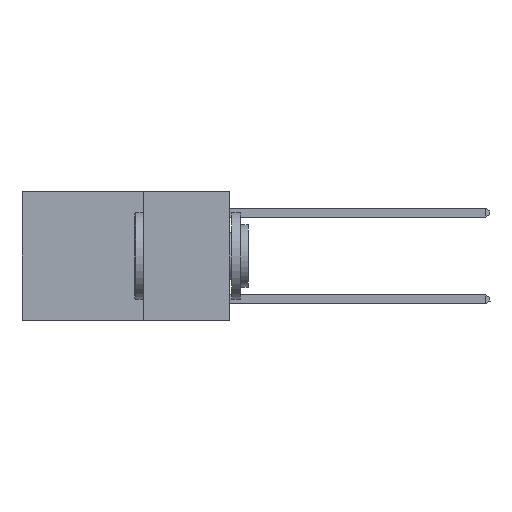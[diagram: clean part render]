
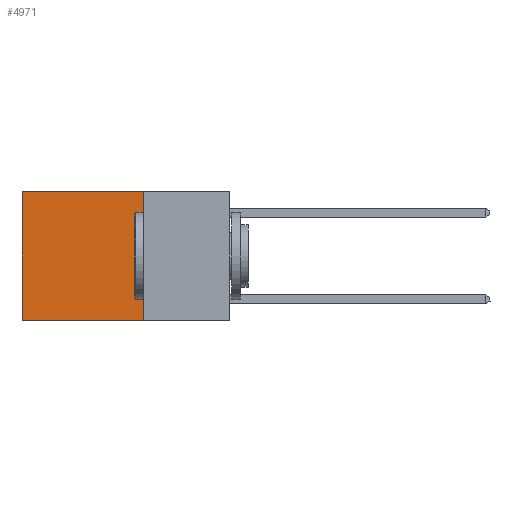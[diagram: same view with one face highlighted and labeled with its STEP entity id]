
A CAD part, left-side view. The second image highlights one B-rep face of the part: STEP entity #4971.
In plain terms, the highlighted planar face has unit normal (-1, 0, 0).
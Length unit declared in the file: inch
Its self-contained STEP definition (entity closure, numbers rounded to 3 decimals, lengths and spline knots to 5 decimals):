
#1460 = LINE ( 'NONE', #19695, #10161 ) ;
#1607 = CARTESIAN_POINT ( 'NONE',  ( 0.2625, 0.6, 0. ) ) ;
#2609 = DIRECTION ( 'NONE',  ( 1., 0., 0. ) ) ;
#2805 = VERTEX_POINT ( 'NONE', #18746 ) ;
#3297 = CARTESIAN_POINT ( 'NONE',  ( 0.2625, 0.25, -0.37 ) ) ;
#4663 = ORIENTED_EDGE ( 'NONE', *, *, #7768, .F. ) ;
#4971 = ADVANCED_FACE ( 'NONE', ( #6856 ), #11848, .F. ) ;
#6209 = CARTESIAN_POINT ( 'NONE',  ( 0.2625, 0.25, 0. ) ) ;
#6226 = EDGE_CURVE ( 'NONE', #7018, #2805, #1460, .T. ) ;
#6318 = EDGE_CURVE ( 'NONE', #17139, #7018, #11827, .T. ) ;
#6856 = FACE_OUTER_BOUND ( 'NONE', #14756, .T. ) ;
#7018 = VERTEX_POINT ( 'NONE', #1607 ) ;
#7043 = ORIENTED_EDGE ( 'NONE', *, *, #6226, .T. ) ;
#7204 = VECTOR ( 'NONE', #12561, 39.37008 ) ;
#7697 = DIRECTION ( 'NONE',  ( 0., 1., 0. ) ) ;
#7768 = EDGE_CURVE ( 'NONE', #10440, #2805, #19367, .T. ) ;
#8475 = LINE ( 'NONE', #9124, #17524 ) ;
#9048 = DIRECTION ( 'NONE',  ( 0., 0., -1. ) ) ;
#9124 = CARTESIAN_POINT ( 'NONE',  ( 0.2625, 0.25, 0. ) ) ;
#9620 = AXIS2_PLACEMENT_3D ( 'NONE', #19339, #2609, #13383 ) ;
#10161 = VECTOR ( 'NONE', #9048, 39.37008 ) ;
#10440 = VERTEX_POINT ( 'NONE', #12814 ) ;
#11055 = CARTESIAN_POINT ( 'NONE',  ( 0.2625, 0.25, 0. ) ) ;
#11201 = ORIENTED_EDGE ( 'NONE', *, *, #6318, .T. ) ;
#11827 = LINE ( 'NONE', #6209, #15880 ) ;
#11848 = PLANE ( 'NONE',  #9620 ) ;
#12488 = EDGE_CURVE ( 'NONE', #17139, #10440, #8475, .T. ) ;
#12561 = DIRECTION ( 'NONE',  ( 0., 1., 0. ) ) ;
#12814 = CARTESIAN_POINT ( 'NONE',  ( 0.2625, 0.25, -0.37 ) ) ;
#13383 = DIRECTION ( 'NONE',  ( 0., 0., -1. ) ) ;
#14756 = EDGE_LOOP ( 'NONE', ( #7043, #4663, #16506, #11201 ) ) ;
#15880 = VECTOR ( 'NONE', #7697, 39.37008 ) ;
#16506 = ORIENTED_EDGE ( 'NONE', *, *, #12488, .F. ) ;
#17139 = VERTEX_POINT ( 'NONE', #11055 ) ;
#17524 = VECTOR ( 'NONE', #19758, 39.37008 ) ;
#18746 = CARTESIAN_POINT ( 'NONE',  ( 0.2625, 0.6, -0.37 ) ) ;
#19339 = CARTESIAN_POINT ( 'NONE',  ( 0.2625, 0.25, 0. ) ) ;
#19367 = LINE ( 'NONE', #3297, #7204 ) ;
#19695 = CARTESIAN_POINT ( 'NONE',  ( 0.2625, 0.6, 0. ) ) ;
#19758 = DIRECTION ( 'NONE',  ( 0., 0., -1. ) ) ;
